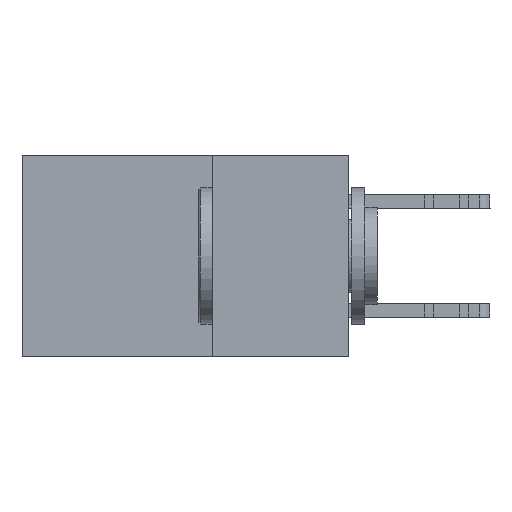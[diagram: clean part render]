
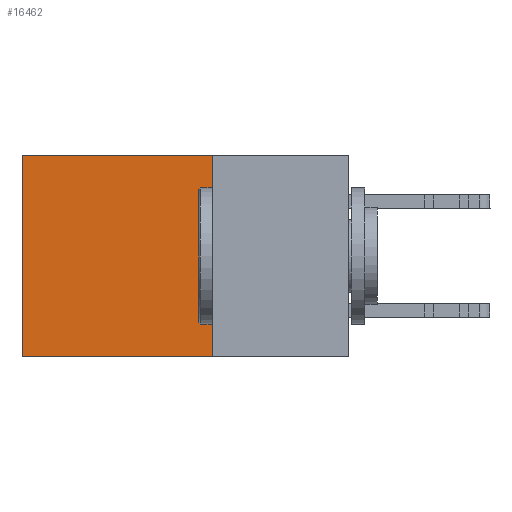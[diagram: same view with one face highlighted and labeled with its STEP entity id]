
A CAD part, left-side view. The second image highlights one B-rep face of the part: STEP entity #16462.
In plain terms, the highlighted planar face has unit normal (-1, 0, 0).
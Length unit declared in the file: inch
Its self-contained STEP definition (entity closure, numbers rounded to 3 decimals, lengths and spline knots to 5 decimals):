
#1118 = EDGE_CURVE ( 'NONE', #15685, #8143, #21987, .T. ) ;
#2958 = VECTOR ( 'NONE', #5861, 39.37008 ) ;
#3136 = PLANE ( 'NONE',  #8258 ) ;
#3534 = CARTESIAN_POINT ( 'NONE',  ( 0.2615, 0.6, -0.37 ) ) ;
#3748 = CARTESIAN_POINT ( 'NONE',  ( 0.2615, 0.25, 0. ) ) ;
#3996 = VERTEX_POINT ( 'NONE', #20179 ) ;
#4341 = VECTOR ( 'NONE', #10452, 39.37008 ) ;
#5201 = CARTESIAN_POINT ( 'NONE',  ( 0.2615, 0.6, 0. ) ) ;
#5861 = DIRECTION ( 'NONE',  ( 0., 0., -1. ) ) ;
#6559 = DIRECTION ( 'NONE',  ( 1., 0., 0. ) ) ;
#6935 = DIRECTION ( 'NONE',  ( 0., 0., -1. ) ) ;
#7281 = ORIENTED_EDGE ( 'NONE', *, *, #17591, .F. ) ;
#7473 = CARTESIAN_POINT ( 'NONE',  ( 0.2615, 0.25, -0.37 ) ) ;
#8143 = VERTEX_POINT ( 'NONE', #5201 ) ;
#8258 = AXIS2_PLACEMENT_3D ( 'NONE', #20411, #6559, #6935 ) ;
#8483 = ORIENTED_EDGE ( 'NONE', *, *, #15880, .F. ) ;
#9969 = EDGE_CURVE ( 'NONE', #8143, #3996, #22957, .T. ) ;
#10452 = DIRECTION ( 'NONE',  ( 0., 1., 0. ) ) ;
#11331 = LINE ( 'NONE', #7473, #13107 ) ;
#12717 = CARTESIAN_POINT ( 'NONE',  ( 0.2615, 0.25, 0. ) ) ;
#13107 = VECTOR ( 'NONE', #21326, 39.37008 ) ;
#13194 = ORIENTED_EDGE ( 'NONE', *, *, #9969, .T. ) ;
#13801 = ORIENTED_EDGE ( 'NONE', *, *, #1118, .T. ) ;
#14337 = EDGE_LOOP ( 'NONE', ( #13194, #7281, #8483, #13801 ) ) ;
#15685 = VERTEX_POINT ( 'NONE', #3748 ) ;
#15880 = EDGE_CURVE ( 'NONE', #15685, #24586, #24924, .T. ) ;
#16299 = VECTOR ( 'NONE', #19163, 39.37008 ) ;
#16462 = ADVANCED_FACE ( 'NONE', ( #20282 ), #3136, .F. ) ;
#17591 = EDGE_CURVE ( 'NONE', #24586, #3996, #11331, .T. ) ;
#19163 = DIRECTION ( 'NONE',  ( 0., 0., -1. ) ) ;
#20179 = CARTESIAN_POINT ( 'NONE',  ( 0.2615, 0.6, -0.37 ) ) ;
#20282 = FACE_OUTER_BOUND ( 'NONE', #14337, .T. ) ;
#20411 = CARTESIAN_POINT ( 'NONE',  ( 0.2615, 0.25, -0.37 ) ) ;
#21326 = DIRECTION ( 'NONE',  ( 0., 1., 0. ) ) ;
#21987 = LINE ( 'NONE', #12717, #4341 ) ;
#22957 = LINE ( 'NONE', #3534, #16299 ) ;
#23010 = CARTESIAN_POINT ( 'NONE',  ( 0.2615, 0.25, -0.37 ) ) ;
#23237 = CARTESIAN_POINT ( 'NONE',  ( 0.2615, 0.25, -0.37 ) ) ;
#24586 = VERTEX_POINT ( 'NONE', #23237 ) ;
#24924 = LINE ( 'NONE', #23010, #2958 ) ;
